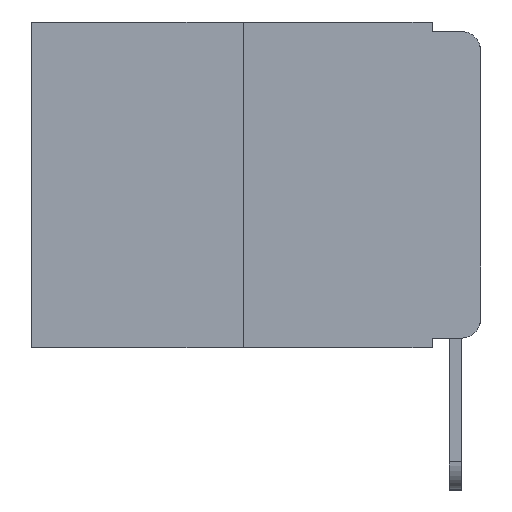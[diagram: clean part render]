
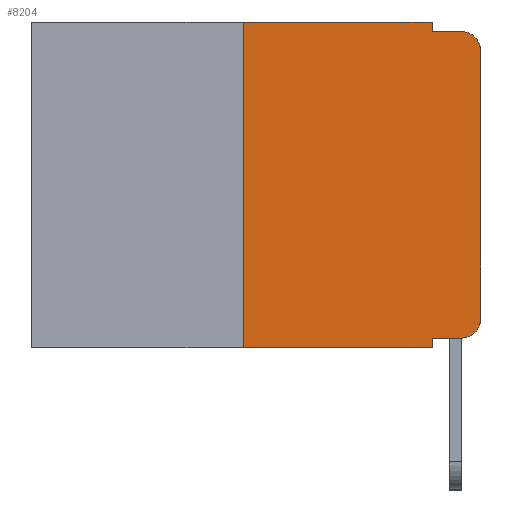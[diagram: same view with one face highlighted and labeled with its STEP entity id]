
A CAD part, left-side view. The second image highlights one B-rep face of the part: STEP entity #8204.
In plain terms, the highlighted planar face has unit normal (-1, 0, 0).
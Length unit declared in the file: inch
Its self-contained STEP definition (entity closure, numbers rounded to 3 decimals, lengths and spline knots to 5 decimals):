
#23 = EDGE_CURVE ( 'NONE', #18384, #3070, #1659, .T. ) ;
#224 = VECTOR ( 'NONE', #15398, 39.37008 ) ;
#559 = DIRECTION ( 'NONE',  ( 0., 0., -1. ) ) ;
#589 = DIRECTION ( 'NONE',  ( 0., 0., -1. ) ) ;
#745 = CIRCLE ( 'NONE', #6840, 0.02 ) ;
#891 = CARTESIAN_POINT ( 'NONE',  ( 0., 0.02, -0.03 ) ) ;
#1096 = VERTEX_POINT ( 'NONE', #15040 ) ;
#1369 = EDGE_CURVE ( 'NONE', #3070, #9484, #10173, .T. ) ;
#1392 = DIRECTION ( 'NONE',  ( 0., -1., 0. ) ) ;
#1573 = CARTESIAN_POINT ( 'NONE',  ( 0., 0.02, -0.313 ) ) ;
#1659 = LINE ( 'NONE', #3893, #19344 ) ;
#1919 = LINE ( 'NONE', #17422, #19052 ) ;
#1942 = FACE_OUTER_BOUND ( 'NONE', #20432, .T. ) ;
#3070 = VERTEX_POINT ( 'NONE', #6649 ) ;
#3456 = DIRECTION ( 'NONE',  ( 0., 0., -1. ) ) ;
#3861 = EDGE_CURVE ( 'NONE', #1096, #9484, #745, .T. ) ;
#3868 = LINE ( 'NONE', #22235, #12575 ) ;
#3893 = CARTESIAN_POINT ( 'NONE',  ( 0., 0.051, 0. ) ) ;
#4172 = EDGE_CURVE ( 'NONE', #19275, #18384, #15209, .T. ) ;
#4173 = DIRECTION ( 'NONE',  ( 1., 0., 0. ) ) ;
#5047 = VERTEX_POINT ( 'NONE', #17468 ) ;
#5088 = EDGE_CURVE ( 'NONE', #18354, #19275, #12343, .T. ) ;
#5498 = DIRECTION ( 'NONE',  ( 0., -1., 0. ) ) ;
#5519 = VECTOR ( 'NONE', #9721, 39.37008 ) ;
#5673 = VECTOR ( 'NONE', #1392, 39.37008 ) ;
#5760 = ORIENTED_EDGE ( 'NONE', *, *, #8647, .T. ) ;
#6306 = EDGE_CURVE ( 'NONE', #21698, #14372, #9851, .T. ) ;
#6649 = CARTESIAN_POINT ( 'NONE',  ( 0., 0.051, -0.01 ) ) ;
#6840 = AXIS2_PLACEMENT_3D ( 'NONE', #891, #8518, #589 ) ;
#6940 = CIRCLE ( 'NONE', #17342, 0.02 ) ;
#8204 = ADVANCED_FACE ( 'NONE', ( #1942 ), #20995, .F. ) ;
#8518 = DIRECTION ( 'NONE',  ( -1., 0., 0. ) ) ;
#8647 = EDGE_CURVE ( 'NONE', #18147, #1096, #1919, .T. ) ;
#9069 = ORIENTED_EDGE ( 'NONE', *, *, #5088, .F. ) ;
#9180 = DIRECTION ( 'NONE',  ( 0., 0., 1. ) ) ;
#9306 = VECTOR ( 'NONE', #12085, 39.37008 ) ;
#9316 = ORIENTED_EDGE ( 'NONE', *, *, #3861, .T. ) ;
#9484 = VERTEX_POINT ( 'NONE', #16390 ) ;
#9629 = CARTESIAN_POINT ( 'NONE',  ( 0., 0., -0.313 ) ) ;
#9721 = DIRECTION ( 'NONE',  ( 0., -1., 0. ) ) ;
#9851 = LINE ( 'NONE', #15284, #9306 ) ;
#10140 = ORIENTED_EDGE ( 'NONE', *, *, #12885, .T. ) ;
#10173 = LINE ( 'NONE', #13220, #5519 ) ;
#10392 = ORIENTED_EDGE ( 'NONE', *, *, #1369, .F. ) ;
#10495 = EDGE_CURVE ( 'NONE', #21698, #5047, #3868, .T. ) ;
#12085 = DIRECTION ( 'NONE',  ( 0., 0., -1. ) ) ;
#12343 = LINE ( 'NONE', #12650, #20562 ) ;
#12359 = CARTESIAN_POINT ( 'NONE',  ( 0., 0.051, -0.343 ) ) ;
#12575 = VECTOR ( 'NONE', #5498, 39.37008 ) ;
#12650 = CARTESIAN_POINT ( 'NONE',  ( 0., 0.25, 0. ) ) ;
#12865 = CARTESIAN_POINT ( 'NONE',  ( 0., 0.051, -0.333 ) ) ;
#12885 = EDGE_CURVE ( 'NONE', #18354, #14372, #18679, .T. ) ;
#12942 = AXIS2_PLACEMENT_3D ( 'NONE', #14444, #4173, #16114 ) ;
#13220 = CARTESIAN_POINT ( 'NONE',  ( 0., 0.051, -0.01 ) ) ;
#13544 = DIRECTION ( 'NONE',  ( 0., 0., 1. ) ) ;
#13763 = DIRECTION ( 'NONE',  ( -1., 0., 0. ) ) ;
#14207 = CARTESIAN_POINT ( 'NONE',  ( 0., 0.473, 0. ) ) ;
#14372 = VERTEX_POINT ( 'NONE', #12359 ) ;
#14444 = CARTESIAN_POINT ( 'NONE',  ( 0., 0.473, 0. ) ) ;
#14502 = ORIENTED_EDGE ( 'NONE', *, *, #10495, .T. ) ;
#15040 = CARTESIAN_POINT ( 'NONE',  ( 0., 0., -0.03 ) ) ;
#15209 = LINE ( 'NONE', #14207, #5673 ) ;
#15284 = CARTESIAN_POINT ( 'NONE',  ( 0., 0.051, 0. ) ) ;
#15398 = DIRECTION ( 'NONE',  ( 0., -1., 0. ) ) ;
#16114 = DIRECTION ( 'NONE',  ( 0., 0., -1. ) ) ;
#16390 = CARTESIAN_POINT ( 'NONE',  ( 0., 0.02, -0.01 ) ) ;
#16657 = CARTESIAN_POINT ( 'NONE',  ( 0., 0.25, -0.343 ) ) ;
#16848 = ORIENTED_EDGE ( 'NONE', *, *, #4172, .F. ) ;
#16998 = CARTESIAN_POINT ( 'NONE',  ( 0., 0.473, -0.343 ) ) ;
#17310 = EDGE_CURVE ( 'NONE', #5047, #18147, #6940, .T. ) ;
#17342 = AXIS2_PLACEMENT_3D ( 'NONE', #1573, #13763, #3456 ) ;
#17422 = CARTESIAN_POINT ( 'NONE',  ( 0., 0., 0. ) ) ;
#17468 = CARTESIAN_POINT ( 'NONE',  ( 0., 0.02, -0.333 ) ) ;
#17783 = ORIENTED_EDGE ( 'NONE', *, *, #17310, .T. ) ;
#17886 = ORIENTED_EDGE ( 'NONE', *, *, #6306, .F. ) ;
#18147 = VERTEX_POINT ( 'NONE', #9629 ) ;
#18354 = VERTEX_POINT ( 'NONE', #16657 ) ;
#18384 = VERTEX_POINT ( 'NONE', #18393 ) ;
#18393 = CARTESIAN_POINT ( 'NONE',  ( 0., 0.051, 0. ) ) ;
#18679 = LINE ( 'NONE', #16998, #224 ) ;
#18776 = CARTESIAN_POINT ( 'NONE',  ( 0., 0.25, 0. ) ) ;
#19052 = VECTOR ( 'NONE', #9180, 39.37008 ) ;
#19275 = VERTEX_POINT ( 'NONE', #18776 ) ;
#19344 = VECTOR ( 'NONE', #559, 39.37008 ) ;
#20432 = EDGE_LOOP ( 'NONE', ( #5760, #9316, #10392, #21706, #16848, #9069, #10140, #17886, #14502, #17783 ) ) ;
#20562 = VECTOR ( 'NONE', #13544, 39.37008 ) ;
#20995 = PLANE ( 'NONE',  #12942 ) ;
#21698 = VERTEX_POINT ( 'NONE', #12865 ) ;
#21706 = ORIENTED_EDGE ( 'NONE', *, *, #23, .F. ) ;
#22235 = CARTESIAN_POINT ( 'NONE',  ( 0., 0.051, -0.333 ) ) ;
